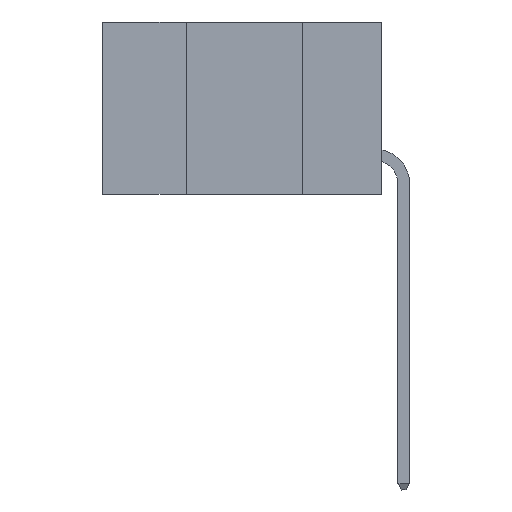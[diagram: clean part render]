
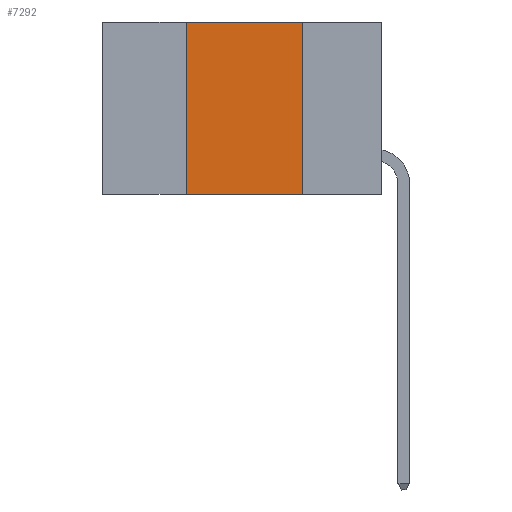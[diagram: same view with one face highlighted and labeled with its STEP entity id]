
A CAD part, left-side view. The second image highlights one B-rep face of the part: STEP entity #7292.
In plain terms, the highlighted planar face has unit normal (-1, 0, 0).
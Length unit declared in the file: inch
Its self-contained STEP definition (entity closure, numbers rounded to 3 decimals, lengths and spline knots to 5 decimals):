
#244 = DIRECTION ( 'NONE',  ( 0., -1., 0. ) ) ;
#286 = DIRECTION ( 'NONE',  ( 0., -1., 0. ) ) ;
#702 = CARTESIAN_POINT ( 'NONE',  ( 0., 0.42, -0.37 ) ) ;
#825 = EDGE_CURVE ( 'NONE', #9981, #3941, #9559, .T. ) ;
#1084 = ORIENTED_EDGE ( 'NONE', *, *, #5042, .F. ) ;
#2154 = EDGE_LOOP ( 'NONE', ( #6142, #1084, #4104, #12207 ) ) ;
#2227 = VERTEX_POINT ( 'NONE', #7636 ) ;
#3053 = CARTESIAN_POINT ( 'NONE',  ( 0., 0.42, 0. ) ) ;
#3691 = CARTESIAN_POINT ( 'NONE',  ( 0., 0.42, 0. ) ) ;
#3941 = VERTEX_POINT ( 'NONE', #8574 ) ;
#4037 = DIRECTION ( 'NONE',  ( 0., 0., -1. ) ) ;
#4104 = ORIENTED_EDGE ( 'NONE', *, *, #7337, .F. ) ;
#4997 = EDGE_CURVE ( 'NONE', #2227, #3941, #11077, .T. ) ;
#4998 = CARTESIAN_POINT ( 'NONE',  ( 0., 0.6, 0. ) ) ;
#5042 = EDGE_CURVE ( 'NONE', #12116, #2227, #10762, .T. ) ;
#5676 = VECTOR ( 'NONE', #7297, 39.37008 ) ;
#6097 = DIRECTION ( 'NONE',  ( 0., 0., 1. ) ) ;
#6142 = ORIENTED_EDGE ( 'NONE', *, *, #4997, .F. ) ;
#6205 = CARTESIAN_POINT ( 'NONE',  ( 0., 0.17, 0. ) ) ;
#6392 = LINE ( 'NONE', #3053, #11491 ) ;
#6719 = FACE_OUTER_BOUND ( 'NONE', #2154, .T. ) ;
#6870 = VECTOR ( 'NONE', #286, 39.37008 ) ;
#7010 = PLANE ( 'NONE',  #10380 ) ;
#7292 = ADVANCED_FACE ( 'NONE', ( #6719 ), #7010, .F. ) ;
#7297 = DIRECTION ( 'NONE',  ( 0., 0., -1. ) ) ;
#7337 = EDGE_CURVE ( 'NONE', #9981, #12116, #6392, .T. ) ;
#7636 = CARTESIAN_POINT ( 'NONE',  ( 0., 0.17, 0. ) ) ;
#8574 = CARTESIAN_POINT ( 'NONE',  ( 0., 0.17, -0.37 ) ) ;
#9559 = LINE ( 'NONE', #13094, #6870 ) ;
#9981 = VERTEX_POINT ( 'NONE', #702 ) ;
#10087 = DIRECTION ( 'NONE',  ( 1., 0., 0. ) ) ;
#10370 = CARTESIAN_POINT ( 'NONE',  ( 0., 0.6, 0. ) ) ;
#10380 = AXIS2_PLACEMENT_3D ( 'NONE', #4998, #10087, #4037 ) ;
#10762 = LINE ( 'NONE', #10370, #13213 ) ;
#11077 = LINE ( 'NONE', #6205, #5676 ) ;
#11491 = VECTOR ( 'NONE', #6097, 39.37008 ) ;
#12116 = VERTEX_POINT ( 'NONE', #3691 ) ;
#12207 = ORIENTED_EDGE ( 'NONE', *, *, #825, .T. ) ;
#13094 = CARTESIAN_POINT ( 'NONE',  ( 0., 0.6, -0.37 ) ) ;
#13213 = VECTOR ( 'NONE', #244, 39.37008 ) ;
